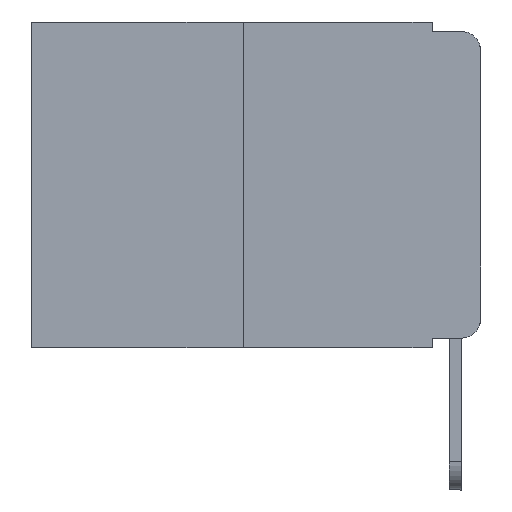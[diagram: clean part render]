
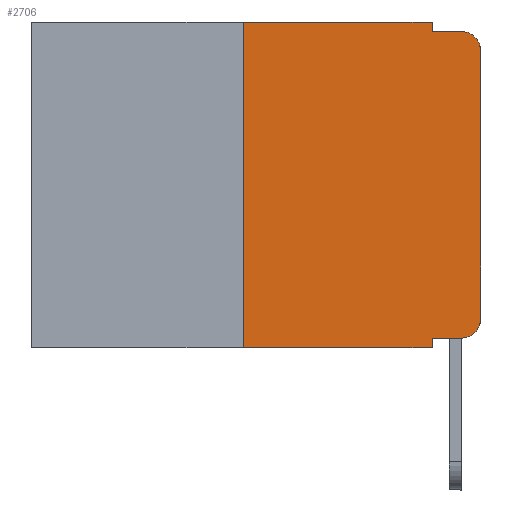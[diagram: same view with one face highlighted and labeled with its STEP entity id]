
A CAD part, left-side view. The second image highlights one B-rep face of the part: STEP entity #2706.
In plain terms, the highlighted planar face has unit normal (-1, 0, 0).
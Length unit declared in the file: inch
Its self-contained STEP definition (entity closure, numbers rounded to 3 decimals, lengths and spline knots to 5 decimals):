
#610 = DIRECTION ( 'NONE',  ( 0., 0., 1. ) ) ;
#671 = VECTOR ( 'NONE', #18406, 39.37008 ) ;
#957 = CARTESIAN_POINT ( 'NONE',  ( 0., 0.051, 0. ) ) ;
#960 = CARTESIAN_POINT ( 'NONE',  ( 0., 0.051, -0.343 ) ) ;
#1010 = CARTESIAN_POINT ( 'NONE',  ( 0., 0.051, 0. ) ) ;
#1334 = ORIENTED_EDGE ( 'NONE', *, *, #21513, .T. ) ;
#1438 = EDGE_CURVE ( 'NONE', #19500, #22297, #16712, .T. ) ;
#1536 = CIRCLE ( 'NONE', #6475, 0.02 ) ;
#1735 = CARTESIAN_POINT ( 'NONE',  ( 0., 0.02, -0.03 ) ) ;
#1854 = CARTESIAN_POINT ( 'NONE',  ( 0., 0.02, -0.333 ) ) ;
#2383 = DIRECTION ( 'NONE',  ( 0., -1., 0. ) ) ;
#2439 = EDGE_CURVE ( 'NONE', #5924, #9941, #12767, .T. ) ;
#2706 = ADVANCED_FACE ( 'NONE', ( #21699 ), #3925, .F. ) ;
#3925 = PLANE ( 'NONE',  #7416 ) ;
#4052 = DIRECTION ( 'NONE',  ( 0., 0., -1. ) ) ;
#4336 = EDGE_CURVE ( 'NONE', #19500, #12980, #6599, .T. ) ;
#4628 = ORIENTED_EDGE ( 'NONE', *, *, #2439, .F. ) ;
#5590 = VECTOR ( 'NONE', #23642, 39.37008 ) ;
#5730 = LINE ( 'NONE', #17933, #5590 ) ;
#5924 = VERTEX_POINT ( 'NONE', #1010 ) ;
#6070 = CARTESIAN_POINT ( 'NONE',  ( 0., 0., 0. ) ) ;
#6137 = CARTESIAN_POINT ( 'NONE',  ( 0., 0.473, 0. ) ) ;
#6475 = AXIS2_PLACEMENT_3D ( 'NONE', #1735, #9663, #13545 ) ;
#6590 = DIRECTION ( 'NONE',  ( 0., -1., 0. ) ) ;
#6599 = LINE ( 'NONE', #16326, #671 ) ;
#6773 = ORIENTED_EDGE ( 'NONE', *, *, #14044, .T. ) ;
#6928 = DIRECTION ( 'NONE',  ( 0., -1., 0. ) ) ;
#7015 = CIRCLE ( 'NONE', #9538, 0.02 ) ;
#7164 = VERTEX_POINT ( 'NONE', #11528 ) ;
#7416 = AXIS2_PLACEMENT_3D ( 'NONE', #13920, #21829, #4052 ) ;
#7449 = DIRECTION ( 'NONE',  ( 0., 0., -1. ) ) ;
#7452 = CARTESIAN_POINT ( 'NONE',  ( 0., 0.02, -0.313 ) ) ;
#7497 = ORIENTED_EDGE ( 'NONE', *, *, #10635, .F. ) ;
#7781 = EDGE_CURVE ( 'NONE', #12980, #5924, #23927, .T. ) ;
#7864 = ORIENTED_EDGE ( 'NONE', *, *, #22524, .T. ) ;
#8128 = VERTEX_POINT ( 'NONE', #1854 ) ;
#8562 = CARTESIAN_POINT ( 'NONE',  ( 0., 0.473, -0.343 ) ) ;
#8564 = CARTESIAN_POINT ( 'NONE',  ( 0., 0.051, -0.333 ) ) ;
#8661 = CARTESIAN_POINT ( 'NONE',  ( 0., 0.051, -0.01 ) ) ;
#9402 = DIRECTION ( 'NONE',  ( 0., 0., -1. ) ) ;
#9538 = AXIS2_PLACEMENT_3D ( 'NONE', #7452, #15347, #9402 ) ;
#9663 = DIRECTION ( 'NONE',  ( -1., 0., 0. ) ) ;
#9941 = VERTEX_POINT ( 'NONE', #8661 ) ;
#10635 = EDGE_CURVE ( 'NONE', #24477, #22297, #5730, .T. ) ;
#10800 = EDGE_LOOP ( 'NONE', ( #6773, #17772, #23762, #4628, #14014, #18888, #10866, #7497, #1334, #7864 ) ) ;
#10866 = ORIENTED_EDGE ( 'NONE', *, *, #1438, .T. ) ;
#11528 = CARTESIAN_POINT ( 'NONE',  ( 0., 0., -0.03 ) ) ;
#11772 = EDGE_CURVE ( 'NONE', #7164, #22869, #1536, .T. ) ;
#12582 = LINE ( 'NONE', #8564, #15273 ) ;
#12767 = LINE ( 'NONE', #957, #24965 ) ;
#12950 = CARTESIAN_POINT ( 'NONE',  ( 0., 0.25, 0. ) ) ;
#12980 = VERTEX_POINT ( 'NONE', #12950 ) ;
#13332 = VERTEX_POINT ( 'NONE', #17012 ) ;
#13545 = DIRECTION ( 'NONE',  ( 0., 0., -1. ) ) ;
#13920 = CARTESIAN_POINT ( 'NONE',  ( 0., 0.473, 0. ) ) ;
#14014 = ORIENTED_EDGE ( 'NONE', *, *, #7781, .F. ) ;
#14044 = EDGE_CURVE ( 'NONE', #13332, #7164, #23860, .T. ) ;
#15273 = VECTOR ( 'NONE', #20482, 39.37008 ) ;
#15347 = DIRECTION ( 'NONE',  ( -1., 0., 0. ) ) ;
#16326 = CARTESIAN_POINT ( 'NONE',  ( 0., 0.25, 0. ) ) ;
#16634 = VECTOR ( 'NONE', #6590, 39.37008 ) ;
#16712 = LINE ( 'NONE', #8562, #16634 ) ;
#16915 = CARTESIAN_POINT ( 'NONE',  ( 0., 0.051, -0.01 ) ) ;
#17012 = CARTESIAN_POINT ( 'NONE',  ( 0., 0., -0.313 ) ) ;
#17772 = ORIENTED_EDGE ( 'NONE', *, *, #11772, .T. ) ;
#17933 = CARTESIAN_POINT ( 'NONE',  ( 0., 0.051, 0. ) ) ;
#18036 = EDGE_CURVE ( 'NONE', #9941, #22869, #24702, .T. ) ;
#18406 = DIRECTION ( 'NONE',  ( 0., 0., 1. ) ) ;
#18888 = ORIENTED_EDGE ( 'NONE', *, *, #4336, .F. ) ;
#19500 = VERTEX_POINT ( 'NONE', #24421 ) ;
#19789 = VECTOR ( 'NONE', #610, 39.37008 ) ;
#20482 = DIRECTION ( 'NONE',  ( 0., -1., 0. ) ) ;
#20819 = VECTOR ( 'NONE', #2383, 39.37008 ) ;
#21019 = CARTESIAN_POINT ( 'NONE',  ( 0., 0.02, -0.01 ) ) ;
#21513 = EDGE_CURVE ( 'NONE', #24477, #8128, #12582, .T. ) ;
#21699 = FACE_OUTER_BOUND ( 'NONE', #10800, .T. ) ;
#21829 = DIRECTION ( 'NONE',  ( 1., 0., 0. ) ) ;
#22219 = VECTOR ( 'NONE', #6928, 39.37008 ) ;
#22297 = VERTEX_POINT ( 'NONE', #960 ) ;
#22438 = CARTESIAN_POINT ( 'NONE',  ( 0., 0.051, -0.333 ) ) ;
#22524 = EDGE_CURVE ( 'NONE', #8128, #13332, #7015, .T. ) ;
#22869 = VERTEX_POINT ( 'NONE', #21019 ) ;
#23642 = DIRECTION ( 'NONE',  ( 0., 0., -1. ) ) ;
#23762 = ORIENTED_EDGE ( 'NONE', *, *, #18036, .F. ) ;
#23860 = LINE ( 'NONE', #6070, #19789 ) ;
#23927 = LINE ( 'NONE', #6137, #20819 ) ;
#24421 = CARTESIAN_POINT ( 'NONE',  ( 0., 0.25, -0.343 ) ) ;
#24477 = VERTEX_POINT ( 'NONE', #22438 ) ;
#24702 = LINE ( 'NONE', #16915, #22219 ) ;
#24965 = VECTOR ( 'NONE', #7449, 39.37008 ) ;
